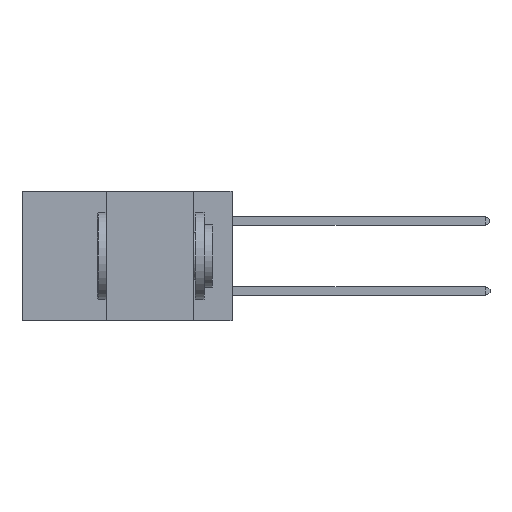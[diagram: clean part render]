
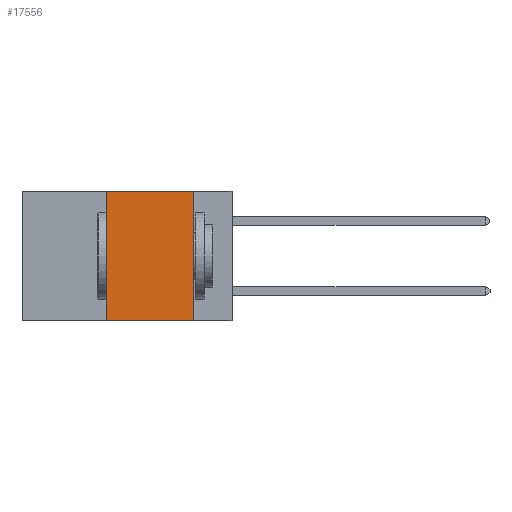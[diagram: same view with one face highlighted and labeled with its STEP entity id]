
A CAD part, left-side view. The second image highlights one B-rep face of the part: STEP entity #17556.
In plain terms, the highlighted planar face has unit normal (-1, 0, 0).
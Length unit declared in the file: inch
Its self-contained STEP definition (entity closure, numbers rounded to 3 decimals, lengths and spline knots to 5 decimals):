
#1284 = DIRECTION ( 'NONE',  ( 0., -1., 0. ) ) ;
#1556 = DIRECTION ( 'NONE',  ( 0., 0., -1. ) ) ;
#1636 = CARTESIAN_POINT ( 'NONE',  ( 0., 0.11, 0. ) ) ;
#2702 = EDGE_CURVE ( 'NONE', #13758, #13124, #3890, .T. ) ;
#2867 = LINE ( 'NONE', #12139, #12555 ) ;
#2971 = CARTESIAN_POINT ( 'NONE',  ( 0., 0.11, -0.37 ) ) ;
#3402 = CARTESIAN_POINT ( 'NONE',  ( 0., 0.6, 0. ) ) ;
#3723 = FACE_OUTER_BOUND ( 'NONE', #20230, .T. ) ;
#3890 = LINE ( 'NONE', #3402, #13280 ) ;
#4255 = DIRECTION ( 'NONE',  ( 0., -1., 0. ) ) ;
#5600 = DIRECTION ( 'NONE',  ( 1., 0., 0. ) ) ;
#5765 = DIRECTION ( 'NONE',  ( 0., 0., -1. ) ) ;
#5836 = CARTESIAN_POINT ( 'NONE',  ( 0., 0.6, 0. ) ) ;
#5963 = EDGE_CURVE ( 'NONE', #13124, #8884, #24755, .T. ) ;
#7441 = VECTOR ( 'NONE', #20231, 39.37008 ) ;
#8884 = VERTEX_POINT ( 'NONE', #2971 ) ;
#9111 = EDGE_CURVE ( 'NONE', #16848, #13758, #14758, .T. ) ;
#12139 = CARTESIAN_POINT ( 'NONE',  ( 0., 0.6, -0.37 ) ) ;
#12505 = EDGE_CURVE ( 'NONE', #16848, #8884, #2867, .T. ) ;
#12555 = VECTOR ( 'NONE', #4255, 39.37008 ) ;
#12711 = ORIENTED_EDGE ( 'NONE', *, *, #9111, .F. ) ;
#13124 = VERTEX_POINT ( 'NONE', #15601 ) ;
#13280 = VECTOR ( 'NONE', #1284, 39.37008 ) ;
#13651 = ORIENTED_EDGE ( 'NONE', *, *, #2702, .F. ) ;
#13758 = VERTEX_POINT ( 'NONE', #17814 ) ;
#14758 = LINE ( 'NONE', #16515, #7441 ) ;
#15601 = CARTESIAN_POINT ( 'NONE',  ( 0., 0.11, 0. ) ) ;
#16515 = CARTESIAN_POINT ( 'NONE',  ( 0., 0.36, 0. ) ) ;
#16848 = VERTEX_POINT ( 'NONE', #22958 ) ;
#17433 = PLANE ( 'NONE',  #21732 ) ;
#17556 = ADVANCED_FACE ( 'NONE', ( #3723 ), #17433, .F. ) ;
#17814 = CARTESIAN_POINT ( 'NONE',  ( 0., 0.36, 0. ) ) ;
#19534 = VECTOR ( 'NONE', #1556, 39.37008 ) ;
#20230 = EDGE_LOOP ( 'NONE', ( #23885, #13651, #12711, #20365 ) ) ;
#20231 = DIRECTION ( 'NONE',  ( 0., 0., 1. ) ) ;
#20365 = ORIENTED_EDGE ( 'NONE', *, *, #12505, .T. ) ;
#21732 = AXIS2_PLACEMENT_3D ( 'NONE', #5836, #5600, #5765 ) ;
#22958 = CARTESIAN_POINT ( 'NONE',  ( 0., 0.36, -0.37 ) ) ;
#23885 = ORIENTED_EDGE ( 'NONE', *, *, #5963, .F. ) ;
#24755 = LINE ( 'NONE', #1636, #19534 ) ;
